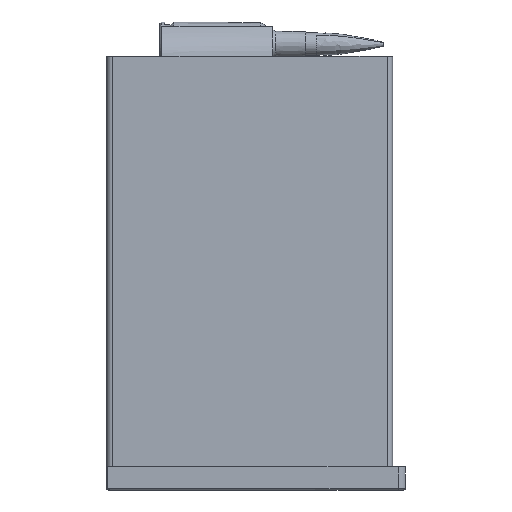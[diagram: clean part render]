
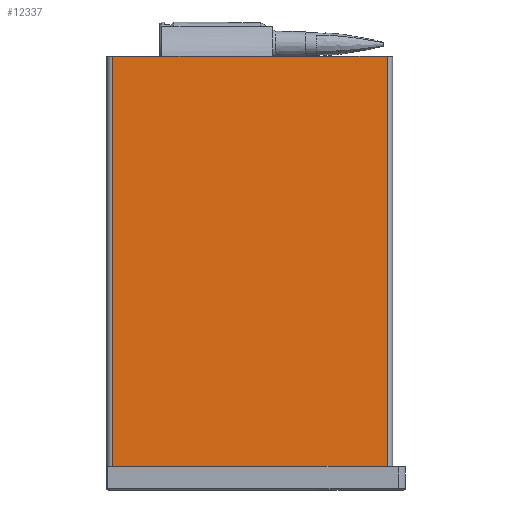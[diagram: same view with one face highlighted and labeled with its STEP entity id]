
A CAD part, front view. The second image highlights one B-rep face of the part: STEP entity #12337.
In plain terms, the highlighted planar face has unit normal (0.019, -1, 0).
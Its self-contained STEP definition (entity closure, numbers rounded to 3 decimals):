
#1023=PLANE('',#13003);
#1791=LINE('',#24357,#2927);
#1808=LINE('',#24584,#2944);
#1858=LINE('',#24760,#2994);
#1859=LINE('',#24763,#2995);
#1860=LINE('',#24765,#2996);
#1861=LINE('',#24766,#2997);
#2927=VECTOR('',#14674,10.);
#2944=VECTOR('',#14703,10.);
#2994=VECTOR('',#14793,10.);
#2995=VECTOR('',#14798,30.005);
#2996=VECTOR('',#14799,10.);
#2997=VECTOR('',#14800,10.);
#3963=FACE_OUTER_BOUND('',#4716,.T.);
#4716=EDGE_LOOP('',(#10301,#10302,#10303,#10304,#10305,#10306));
#5906=VERTEX_POINT('',#24354);
#5907=VERTEX_POINT('',#24356);
#5936=VERTEX_POINT('',#24581);
#5937=VERTEX_POINT('',#24583);
#5983=VERTEX_POINT('',#24759);
#5984=VERTEX_POINT('',#24764);
#7396=EDGE_CURVE('',#5906,#5907,#1791,.T.);
#7430=EDGE_CURVE('',#5936,#5937,#1808,.T.);
#7490=EDGE_CURVE('',#5907,#5983,#1858,.T.);
#7492=EDGE_CURVE('',#5906,#5937,#1859,.T.);
#7493=EDGE_CURVE('',#5984,#5936,#1860,.T.);
#7494=EDGE_CURVE('',#5984,#5983,#1861,.T.);
#10301=ORIENTED_EDGE('',*,*,#7490,.F.);
#10302=ORIENTED_EDGE('',*,*,#7396,.F.);
#10303=ORIENTED_EDGE('',*,*,#7492,.T.);
#10304=ORIENTED_EDGE('',*,*,#7430,.F.);
#10305=ORIENTED_EDGE('',*,*,#7493,.F.);
#10306=ORIENTED_EDGE('',*,*,#7494,.T.);
#12337=ADVANCED_FACE('',(#3963),#1023,.T.);
#13003=AXIS2_PLACEMENT_3D('',#24762,#14796,#14797);
#14674=DIRECTION('',(1.,0.019,0.));
#14703=DIRECTION('',(1.,0.019,0.));
#14793=DIRECTION('',(0.,0.,-1.));
#14796=DIRECTION('center_axis',(0.019,-1.,0.));
#14797=DIRECTION('ref_axis',(1.,0.019,0.));
#14798=DIRECTION('',(-1.,-0.019,0.));
#14799=DIRECTION('',(0.,0.,1.));
#14800=DIRECTION('',(1.,0.019,0.));
#24354=CARTESIAN_POINT('',(45.,0.842,115.));
#24356=CARTESIAN_POINT('',(76.028,1.422,115.));
#24357=CARTESIAN_POINT('',(0.,0.,115.));
#24581=CARTESIAN_POINT('',(1.528,0.029,115.));
#24583=CARTESIAN_POINT('',(15.,0.281,115.));
#24584=CARTESIAN_POINT('',(0.,0.,115.));
#24759=CARTESIAN_POINT('',(76.028,1.422,2.));
#24760=CARTESIAN_POINT('',(76.028,1.422,0.));
#24762=CARTESIAN_POINT('Origin',(0.,0.,0.));
#24763=CARTESIAN_POINT('',(45.,0.842,115.));
#24764=CARTESIAN_POINT('',(1.528,0.029,2.));
#24765=CARTESIAN_POINT('',(1.528,0.029,0.));
#24766=CARTESIAN_POINT('',(19.859,0.372,2.));
